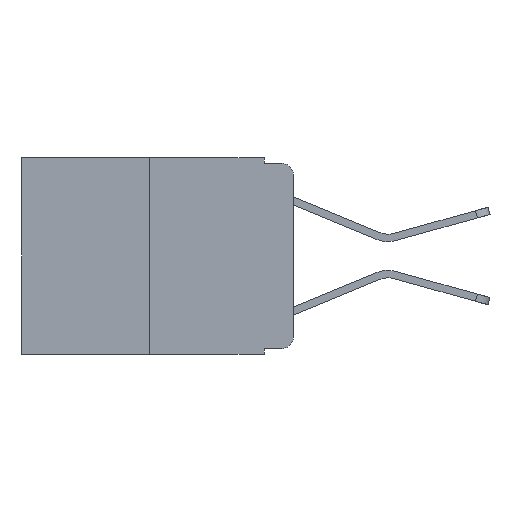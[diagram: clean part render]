
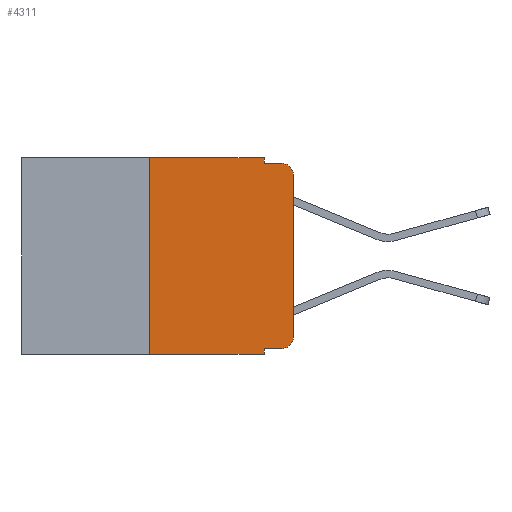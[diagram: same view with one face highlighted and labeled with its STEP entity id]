
A CAD part, left-side view. The second image highlights one B-rep face of the part: STEP entity #4311.
In plain terms, the highlighted planar face has unit normal (-1, 0, 0).
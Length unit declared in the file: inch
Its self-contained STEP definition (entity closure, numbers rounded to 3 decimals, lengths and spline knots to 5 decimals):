
#412 = ORIENTED_EDGE ( 'NONE', *, *, #4944, .F. ) ;
#508 = CARTESIAN_POINT ( 'NONE',  ( 0., 0.051, 0. ) ) ;
#621 = VECTOR ( 'NONE', #19539, 39.37008 ) ;
#684 = CARTESIAN_POINT ( 'NONE',  ( 0., 0.25, 0. ) ) ;
#1199 = DIRECTION ( 'NONE',  ( -1., 0., 0. ) ) ;
#1246 = CARTESIAN_POINT ( 'NONE',  ( 0., 0.473, 0. ) ) ;
#1296 = CARTESIAN_POINT ( 'NONE',  ( 0., 0.02, -0.313 ) ) ;
#1758 = EDGE_CURVE ( 'NONE', #4516, #13602, #19437, .T. ) ;
#2129 = AXIS2_PLACEMENT_3D ( 'NONE', #3182, #13890, #4749 ) ;
#2582 = VERTEX_POINT ( 'NONE', #11638 ) ;
#2695 = VERTEX_POINT ( 'NONE', #17229 ) ;
#2842 = EDGE_CURVE ( 'NONE', #11271, #4516, #4997, .T. ) ;
#3182 = CARTESIAN_POINT ( 'NONE',  ( 0., 0.473, 0. ) ) ;
#3216 = ORIENTED_EDGE ( 'NONE', *, *, #16448, .T. ) ;
#3450 = DIRECTION ( 'NONE',  ( 0., -1., 0. ) ) ;
#3878 = VECTOR ( 'NONE', #15842, 39.37008 ) ;
#3991 = ORIENTED_EDGE ( 'NONE', *, *, #1758, .T. ) ;
#3993 = CARTESIAN_POINT ( 'NONE',  ( 0., 0.25, -0.343 ) ) ;
#4311 = ADVANCED_FACE ( 'NONE', ( #18662 ), #9319, .F. ) ;
#4423 = CARTESIAN_POINT ( 'NONE',  ( 0., 0.25, 0. ) ) ;
#4470 = DIRECTION ( 'NONE',  ( 0., -1., 0. ) ) ;
#4516 = VERTEX_POINT ( 'NONE', #15947 ) ;
#4590 = DIRECTION ( 'NONE',  ( 0., 0., -1. ) ) ;
#4749 = DIRECTION ( 'NONE',  ( 0., 0., -1. ) ) ;
#4777 = ORIENTED_EDGE ( 'NONE', *, *, #18534, .F. ) ;
#4944 = EDGE_CURVE ( 'NONE', #11271, #2582, #19118, .T. ) ;
#4997 = LINE ( 'NONE', #6016, #10027 ) ;
#5047 = LINE ( 'NONE', #16607, #8651 ) ;
#5218 = VERTEX_POINT ( 'NONE', #508 ) ;
#6005 = LINE ( 'NONE', #1246, #14073 ) ;
#6016 = CARTESIAN_POINT ( 'NONE',  ( 0., 0.051, -0.333 ) ) ;
#6021 = EDGE_CURVE ( 'NONE', #12227, #13684, #13049, .T. ) ;
#6457 = CARTESIAN_POINT ( 'NONE',  ( 0., 0., -0.03 ) ) ;
#6870 = DIRECTION ( 'NONE',  ( 0., 0., 1. ) ) ;
#7048 = EDGE_CURVE ( 'NONE', #5218, #2695, #19486, .T. ) ;
#7866 = CARTESIAN_POINT ( 'NONE',  ( 0., 0.02, -0.03 ) ) ;
#8026 = VECTOR ( 'NONE', #6870, 39.37008 ) ;
#8045 = EDGE_CURVE ( 'NONE', #2695, #12535, #5047, .T. ) ;
#8651 = VECTOR ( 'NONE', #4470, 39.37008 ) ;
#9293 = CARTESIAN_POINT ( 'NONE',  ( 0., 0.02, -0.01 ) ) ;
#9319 = PLANE ( 'NONE',  #2129 ) ;
#9332 = ORIENTED_EDGE ( 'NONE', *, *, #8045, .F. ) ;
#9381 = DIRECTION ( 'NONE',  ( 0., 0., -1. ) ) ;
#10027 = VECTOR ( 'NONE', #13887, 39.37008 ) ;
#11083 = EDGE_CURVE ( 'NONE', #15918, #12535, #18430, .T. ) ;
#11193 = ORIENTED_EDGE ( 'NONE', *, *, #12106, .T. ) ;
#11271 = VERTEX_POINT ( 'NONE', #17387 ) ;
#11638 = CARTESIAN_POINT ( 'NONE',  ( 0., 0.051, -0.343 ) ) ;
#11757 = AXIS2_PLACEMENT_3D ( 'NONE', #1296, #1199, #14197 ) ;
#12102 = VECTOR ( 'NONE', #4590, 39.37008 ) ;
#12106 = EDGE_CURVE ( 'NONE', #13602, #15918, #12547, .T. ) ;
#12227 = VERTEX_POINT ( 'NONE', #3993 ) ;
#12535 = VERTEX_POINT ( 'NONE', #9293 ) ;
#12547 = LINE ( 'NONE', #18886, #8026 ) ;
#12714 = CARTESIAN_POINT ( 'NONE',  ( 0., 0.473, -0.343 ) ) ;
#13049 = LINE ( 'NONE', #4423, #621 ) ;
#13131 = LINE ( 'NONE', #12714, #17120 ) ;
#13565 = DIRECTION ( 'NONE',  ( 0., -1., 0. ) ) ;
#13602 = VERTEX_POINT ( 'NONE', #18895 ) ;
#13684 = VERTEX_POINT ( 'NONE', #684 ) ;
#13887 = DIRECTION ( 'NONE',  ( 0., -1., 0. ) ) ;
#13890 = DIRECTION ( 'NONE',  ( 1., 0., 0. ) ) ;
#14073 = VECTOR ( 'NONE', #13565, 39.37008 ) ;
#14197 = DIRECTION ( 'NONE',  ( 0., 0., -1. ) ) ;
#14322 = CARTESIAN_POINT ( 'NONE',  ( 0., 0.051, 0. ) ) ;
#14761 = ORIENTED_EDGE ( 'NONE', *, *, #2842, .T. ) ;
#15267 = CARTESIAN_POINT ( 'NONE',  ( 0., 0.051, 0. ) ) ;
#15842 = DIRECTION ( 'NONE',  ( 0., 0., -1. ) ) ;
#15867 = ORIENTED_EDGE ( 'NONE', *, *, #6021, .F. ) ;
#15918 = VERTEX_POINT ( 'NONE', #6457 ) ;
#15947 = CARTESIAN_POINT ( 'NONE',  ( 0., 0.02, -0.333 ) ) ;
#16448 = EDGE_CURVE ( 'NONE', #12227, #2582, #13131, .T. ) ;
#16607 = CARTESIAN_POINT ( 'NONE',  ( 0., 0.051, -0.01 ) ) ;
#17120 = VECTOR ( 'NONE', #3450, 39.37008 ) ;
#17127 = EDGE_LOOP ( 'NONE', ( #11193, #17142, #9332, #18964, #4777, #15867, #3216, #412, #14761, #3991 ) ) ;
#17142 = ORIENTED_EDGE ( 'NONE', *, *, #11083, .T. ) ;
#17229 = CARTESIAN_POINT ( 'NONE',  ( 0., 0.051, -0.01 ) ) ;
#17334 = AXIS2_PLACEMENT_3D ( 'NONE', #7866, #18396, #9381 ) ;
#17387 = CARTESIAN_POINT ( 'NONE',  ( 0., 0.051, -0.333 ) ) ;
#18396 = DIRECTION ( 'NONE',  ( -1., 0., 0. ) ) ;
#18430 = CIRCLE ( 'NONE', #17334, 0.02 ) ;
#18534 = EDGE_CURVE ( 'NONE', #13684, #5218, #6005, .T. ) ;
#18662 = FACE_OUTER_BOUND ( 'NONE', #17127, .T. ) ;
#18886 = CARTESIAN_POINT ( 'NONE',  ( 0., 0., 0. ) ) ;
#18895 = CARTESIAN_POINT ( 'NONE',  ( 0., 0., -0.313 ) ) ;
#18964 = ORIENTED_EDGE ( 'NONE', *, *, #7048, .F. ) ;
#19118 = LINE ( 'NONE', #15267, #12102 ) ;
#19437 = CIRCLE ( 'NONE', #11757, 0.02 ) ;
#19486 = LINE ( 'NONE', #14322, #3878 ) ;
#19539 = DIRECTION ( 'NONE',  ( 0., 0., 1. ) ) ;
